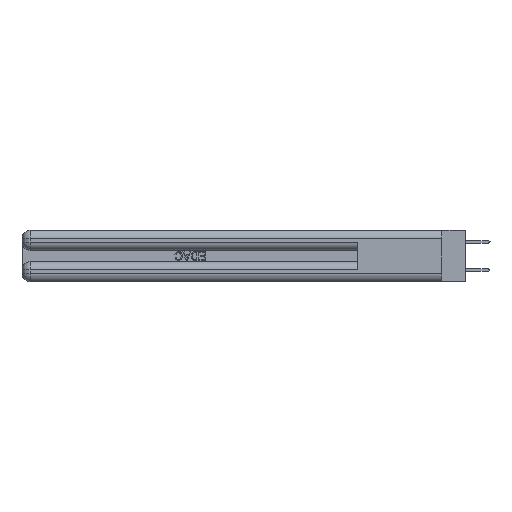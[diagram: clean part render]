
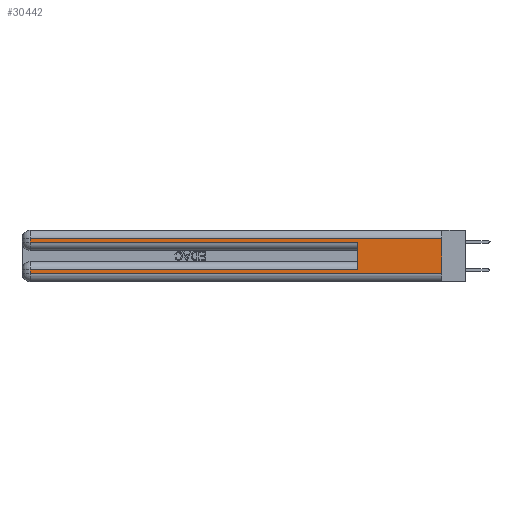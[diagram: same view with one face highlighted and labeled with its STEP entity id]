
A CAD part, left-side view. The second image highlights one B-rep face of the part: STEP entity #30442.
In plain terms, the highlighted planar face has unit normal (-1, 0, 0).
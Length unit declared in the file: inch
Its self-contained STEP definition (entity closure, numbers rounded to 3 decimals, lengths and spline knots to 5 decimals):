
#99 = EDGE_CURVE ( 'NONE', #10188, #5701, #23924, .T. ) ;
#785 = LINE ( 'NONE', #26777, #15869 ) ;
#1978 = EDGE_LOOP ( 'NONE', ( #26320, #8263, #40994, #19602, #13482, #11201, #8091, #39569 ) ) ;
#2972 = VECTOR ( 'NONE', #8870, 39.37008 ) ;
#4207 = DIRECTION ( 'NONE',  ( 0., 1., 0. ) ) ;
#4507 = VERTEX_POINT ( 'NONE', #22294 ) ;
#5701 = VERTEX_POINT ( 'NONE', #31714 ) ;
#6228 = DIRECTION ( 'NONE',  ( 0., 0., 1. ) ) ;
#6587 = CARTESIAN_POINT ( 'NONE',  ( 0., 0., 0.37 ) ) ;
#8091 = ORIENTED_EDGE ( 'NONE', *, *, #99, .T. ) ;
#8263 = ORIENTED_EDGE ( 'NONE', *, *, #26717, .T. ) ;
#8870 = DIRECTION ( 'NONE',  ( 0., -1., 0. ) ) ;
#9406 = DIRECTION ( 'NONE',  ( 1., 0., 0. ) ) ;
#10188 = VERTEX_POINT ( 'NONE', #11121 ) ;
#11121 = CARTESIAN_POINT ( 'NONE',  ( 0., 2.94, 0.085 ) ) ;
#11201 = ORIENTED_EDGE ( 'NONE', *, *, #26721, .T. ) ;
#12538 = LINE ( 'NONE', #24930, #2972 ) ;
#13482 = ORIENTED_EDGE ( 'NONE', *, *, #37244, .F. ) ;
#14412 = CARTESIAN_POINT ( 'NONE',  ( 0., 0.6, 0.285 ) ) ;
#15629 = CARTESIAN_POINT ( 'NONE',  ( 0., 0., 0.285 ) ) ;
#15869 = VECTOR ( 'NONE', #30025, 39.37008 ) ;
#18530 = EDGE_CURVE ( 'NONE', #21720, #33713, #31446, .T. ) ;
#18901 = DIRECTION ( 'NONE',  ( 0., -1., 0. ) ) ;
#19188 = CARTESIAN_POINT ( 'NONE',  ( 0., 2.94, 0.31 ) ) ;
#19397 = VECTOR ( 'NONE', #6228, 39.37008 ) ;
#19602 = ORIENTED_EDGE ( 'NONE', *, *, #18530, .T. ) ;
#19932 = CARTESIAN_POINT ( 'NONE',  ( 0., 0.6, 0.085 ) ) ;
#20211 = LINE ( 'NONE', #23083, #28829 ) ;
#21706 = VERTEX_POINT ( 'NONE', #19188 ) ;
#21720 = VERTEX_POINT ( 'NONE', #38649 ) ;
#22294 = CARTESIAN_POINT ( 'NONE',  ( 0., 0., 0.31 ) ) ;
#22296 = CARTESIAN_POINT ( 'NONE',  ( 0., 0.6, 0.145 ) ) ;
#22655 = DIRECTION ( 'NONE',  ( 0., 0., -1. ) ) ;
#23083 = CARTESIAN_POINT ( 'NONE',  ( 0., 2.94, 0.37 ) ) ;
#23524 = CARTESIAN_POINT ( 'NONE',  ( 0., 0., 0.31 ) ) ;
#23850 = EDGE_CURVE ( 'NONE', #5701, #37879, #12538, .T. ) ;
#23924 = LINE ( 'NONE', #32207, #41075 ) ;
#24516 = VECTOR ( 'NONE', #22655, 39.37008 ) ;
#24930 = CARTESIAN_POINT ( 'NONE',  ( 0., 0., 0.06 ) ) ;
#25299 = EDGE_CURVE ( 'NONE', #4507, #37879, #41637, .T. ) ;
#25479 = PLANE ( 'NONE',  #31428 ) ;
#26320 = ORIENTED_EDGE ( 'NONE', *, *, #25299, .F. ) ;
#26717 = EDGE_CURVE ( 'NONE', #4507, #21706, #35065, .T. ) ;
#26721 = EDGE_CURVE ( 'NONE', #38395, #10188, #785, .T. ) ;
#26777 = CARTESIAN_POINT ( 'NONE',  ( 0., 0., 0.085 ) ) ;
#27997 = LINE ( 'NONE', #22296, #19397 ) ;
#28738 = CARTESIAN_POINT ( 'NONE',  ( 0., 0., 0.37 ) ) ;
#28829 = VECTOR ( 'NONE', #39164, 39.37008 ) ;
#28935 = DIRECTION ( 'NONE',  ( 0., 0., -1. ) ) ;
#30025 = DIRECTION ( 'NONE',  ( 0., 1., 0. ) ) ;
#30442 = ADVANCED_FACE ( 'NONE', ( #38130 ), #25479, .F. ) ;
#31428 = AXIS2_PLACEMENT_3D ( 'NONE', #28738, #9406, #32000 ) ;
#31446 = LINE ( 'NONE', #15629, #38983 ) ;
#31714 = CARTESIAN_POINT ( 'NONE',  ( 0., 2.94, 0.06 ) ) ;
#32000 = DIRECTION ( 'NONE',  ( 0., 0., -1. ) ) ;
#32207 = CARTESIAN_POINT ( 'NONE',  ( 0., 2.94, 0.37 ) ) ;
#33713 = VERTEX_POINT ( 'NONE', #14412 ) ;
#35065 = LINE ( 'NONE', #23524, #41561 ) ;
#36461 = CARTESIAN_POINT ( 'NONE',  ( 0., 0., 0.06 ) ) ;
#37244 = EDGE_CURVE ( 'NONE', #38395, #33713, #27997, .T. ) ;
#37879 = VERTEX_POINT ( 'NONE', #36461 ) ;
#38130 = FACE_OUTER_BOUND ( 'NONE', #1978, .T. ) ;
#38395 = VERTEX_POINT ( 'NONE', #19932 ) ;
#38649 = CARTESIAN_POINT ( 'NONE',  ( 0., 2.94, 0.285 ) ) ;
#38983 = VECTOR ( 'NONE', #18901, 39.37008 ) ;
#39164 = DIRECTION ( 'NONE',  ( 0., 0., -1. ) ) ;
#39569 = ORIENTED_EDGE ( 'NONE', *, *, #23850, .T. ) ;
#40994 = ORIENTED_EDGE ( 'NONE', *, *, #41082, .T. ) ;
#41075 = VECTOR ( 'NONE', #28935, 39.37008 ) ;
#41082 = EDGE_CURVE ( 'NONE', #21706, #21720, #20211, .T. ) ;
#41561 = VECTOR ( 'NONE', #4207, 39.37008 ) ;
#41637 = LINE ( 'NONE', #6587, #24516 ) ;
